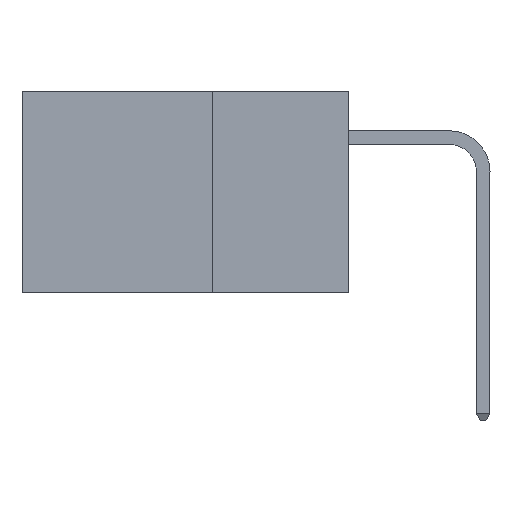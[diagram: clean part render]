
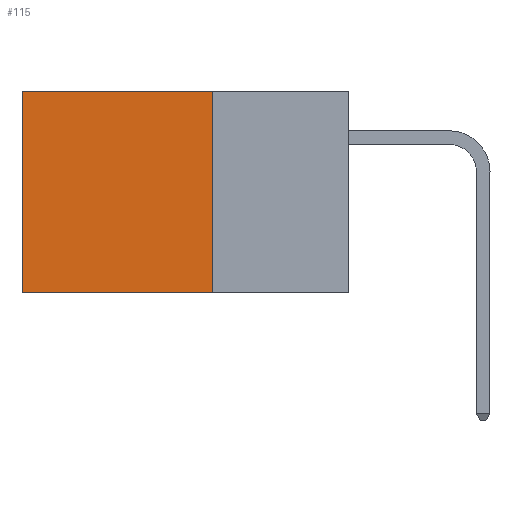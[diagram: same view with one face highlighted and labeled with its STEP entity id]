
A CAD part, left-side view. The second image highlights one B-rep face of the part: STEP entity #115.
In plain terms, the highlighted planar face has unit normal (-1, 0, 0).
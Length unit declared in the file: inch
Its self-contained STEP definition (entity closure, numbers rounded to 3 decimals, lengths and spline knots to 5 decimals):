
#42 = DIRECTION ( 'NONE',  ( 0., 0., -1. ) ) ;
#99 = CARTESIAN_POINT ( 'NONE',  ( 0.2875, 0.25, 0. ) ) ;
#115 = ADVANCED_FACE ( 'NONE', ( #4064 ), #2005, .F. ) ;
#142 = VERTEX_POINT ( 'NONE', #788 ) ;
#416 = LINE ( 'NONE', #99, #9071 ) ;
#509 = CARTESIAN_POINT ( 'NONE',  ( 0.2875, 0.6, -0.37 ) ) ;
#788 = CARTESIAN_POINT ( 'NONE',  ( 0.2875, 0.25, 0. ) ) ;
#1287 = LINE ( 'NONE', #12771, #3913 ) ;
#1426 = CARTESIAN_POINT ( 'NONE',  ( 0.2875, 0.25, -0.37 ) ) ;
#1770 = CARTESIAN_POINT ( 'NONE',  ( 0.2875, 0.25, -0.37 ) ) ;
#1834 = DIRECTION ( 'NONE',  ( 0., 0., -1. ) ) ;
#1851 = DIRECTION ( 'NONE',  ( 1., 0., 0. ) ) ;
#1868 = CARTESIAN_POINT ( 'NONE',  ( 0.2875, 0.25, 0. ) ) ;
#2005 = PLANE ( 'NONE',  #10084 ) ;
#2981 = DIRECTION ( 'NONE',  ( 0., 0., -1. ) ) ;
#3199 = LINE ( 'NONE', #1426, #6144 ) ;
#3913 = VECTOR ( 'NONE', #5546, 39.37008 ) ;
#4064 = FACE_OUTER_BOUND ( 'NONE', #8106, .T. ) ;
#4389 = ORIENTED_EDGE ( 'NONE', *, *, #10537, .T. ) ;
#4489 = ORIENTED_EDGE ( 'NONE', *, *, #13139, .F. ) ;
#4546 = ORIENTED_EDGE ( 'NONE', *, *, #6455, .F. ) ;
#4572 = ORIENTED_EDGE ( 'NONE', *, *, #13617, .T. ) ;
#4940 = VERTEX_POINT ( 'NONE', #5788 ) ;
#5546 = DIRECTION ( 'NONE',  ( 0., 1., 0. ) ) ;
#5788 = CARTESIAN_POINT ( 'NONE',  ( 0.2875, 0.6, 0. ) ) ;
#6144 = VECTOR ( 'NONE', #7948, 39.37008 ) ;
#6455 = EDGE_CURVE ( 'NONE', #142, #8285, #416, .T. ) ;
#7948 = DIRECTION ( 'NONE',  ( 0., 1., 0. ) ) ;
#8106 = EDGE_LOOP ( 'NONE', ( #4389, #4489, #4546, #4572 ) ) ;
#8285 = VERTEX_POINT ( 'NONE', #1770 ) ;
#9071 = VECTOR ( 'NONE', #42, 39.37008 ) ;
#10084 = AXIS2_PLACEMENT_3D ( 'NONE', #1868, #1851, #1834 ) ;
#10472 = CARTESIAN_POINT ( 'NONE',  ( 0.2875, 0.6, 0. ) ) ;
#10537 = EDGE_CURVE ( 'NONE', #4940, #11713, #12483, .T. ) ;
#11713 = VERTEX_POINT ( 'NONE', #509 ) ;
#12483 = LINE ( 'NONE', #10472, #13137 ) ;
#12771 = CARTESIAN_POINT ( 'NONE',  ( 0.2875, 0.25, 0. ) ) ;
#13137 = VECTOR ( 'NONE', #2981, 39.37008 ) ;
#13139 = EDGE_CURVE ( 'NONE', #8285, #11713, #3199, .T. ) ;
#13617 = EDGE_CURVE ( 'NONE', #142, #4940, #1287, .T. ) ;
